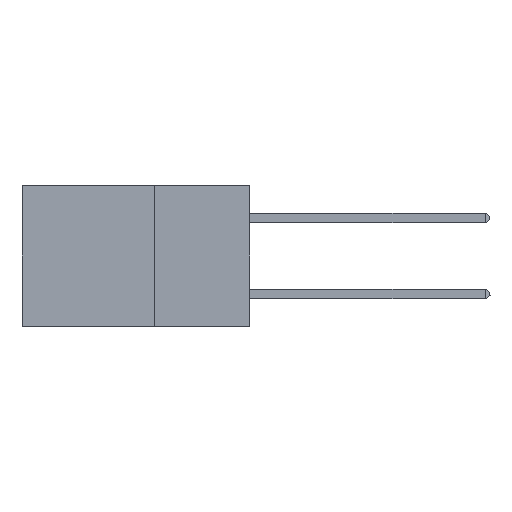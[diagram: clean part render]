
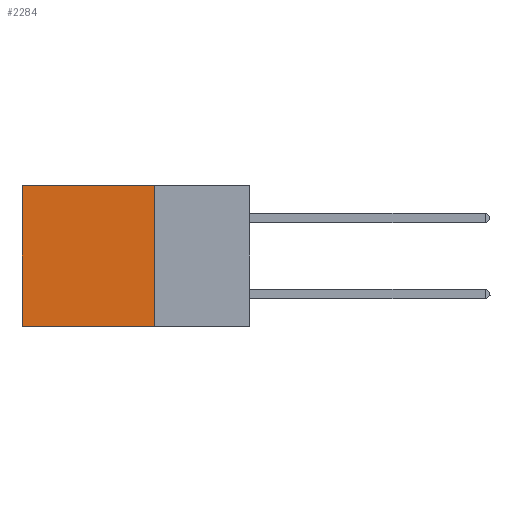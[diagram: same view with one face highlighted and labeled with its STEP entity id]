
A CAD part, left-side view. The second image highlights one B-rep face of the part: STEP entity #2284.
In plain terms, the highlighted planar face has unit normal (-1, 0, 0).
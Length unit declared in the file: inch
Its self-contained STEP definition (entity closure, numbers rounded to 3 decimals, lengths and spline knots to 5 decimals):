
#1475 = DIRECTION ( 'NONE',  ( 0., 0., -1. ) ) ;
#2284 = ADVANCED_FACE ( 'NONE', ( #34359 ), #17217, .F. ) ;
#2665 = AXIS2_PLACEMENT_3D ( 'NONE', #16799, #23824, #33829 ) ;
#2701 = DIRECTION ( 'NONE',  ( 0., 0., -1. ) ) ;
#3450 = CARTESIAN_POINT ( 'NONE',  ( 0.2875, 0.25, 0. ) ) ;
#3699 = LINE ( 'NONE', #32307, #22293 ) ;
#4360 = ORIENTED_EDGE ( 'NONE', *, *, #36327, .F. ) ;
#6196 = VERTEX_POINT ( 'NONE', #22039 ) ;
#8062 = VERTEX_POINT ( 'NONE', #24299 ) ;
#9251 = VECTOR ( 'NONE', #2701, 39.37008 ) ;
#10773 = LINE ( 'NONE', #39113, #9251 ) ;
#13181 = DIRECTION ( 'NONE',  ( 0., 1., 0. ) ) ;
#13302 = LINE ( 'NONE', #18218, #26184 ) ;
#13500 = VERTEX_POINT ( 'NONE', #3450 ) ;
#15913 = ORIENTED_EDGE ( 'NONE', *, *, #26204, .T. ) ;
#16799 = CARTESIAN_POINT ( 'NONE',  ( 0.2875, 0.25, 0. ) ) ;
#17217 = PLANE ( 'NONE',  #2665 ) ;
#17249 = ORIENTED_EDGE ( 'NONE', *, *, #39795, .F. ) ;
#18218 = CARTESIAN_POINT ( 'NONE',  ( 0.2875, 0.25, 0. ) ) ;
#20271 = ORIENTED_EDGE ( 'NONE', *, *, #29562, .T. ) ;
#20923 = EDGE_LOOP ( 'NONE', ( #15913, #4360, #17249, #20271 ) ) ;
#21085 = VERTEX_POINT ( 'NONE', #25900 ) ;
#22039 = CARTESIAN_POINT ( 'NONE',  ( 0.2875, 0.6, -0.37 ) ) ;
#22171 = DIRECTION ( 'NONE',  ( 0., 1., 0. ) ) ;
#22293 = VECTOR ( 'NONE', #22171, 39.37008 ) ;
#23645 = CARTESIAN_POINT ( 'NONE',  ( 0.2875, 0.25, 0. ) ) ;
#23824 = DIRECTION ( 'NONE',  ( 1., 0., 0. ) ) ;
#24299 = CARTESIAN_POINT ( 'NONE',  ( 0.2875, 0.6, 0. ) ) ;
#25900 = CARTESIAN_POINT ( 'NONE',  ( 0.2875, 0.25, -0.37 ) ) ;
#26184 = VECTOR ( 'NONE', #1475, 39.37008 ) ;
#26204 = EDGE_CURVE ( 'NONE', #8062, #6196, #10773, .T. ) ;
#29562 = EDGE_CURVE ( 'NONE', #13500, #8062, #42004, .T. ) ;
#32307 = CARTESIAN_POINT ( 'NONE',  ( 0.2875, 0.25, -0.37 ) ) ;
#33266 = VECTOR ( 'NONE', #13181, 39.37008 ) ;
#33829 = DIRECTION ( 'NONE',  ( 0., 0., -1. ) ) ;
#34359 = FACE_OUTER_BOUND ( 'NONE', #20923, .T. ) ;
#36327 = EDGE_CURVE ( 'NONE', #21085, #6196, #3699, .T. ) ;
#39113 = CARTESIAN_POINT ( 'NONE',  ( 0.2875, 0.6, 0. ) ) ;
#39795 = EDGE_CURVE ( 'NONE', #13500, #21085, #13302, .T. ) ;
#42004 = LINE ( 'NONE', #23645, #33266 ) ;
